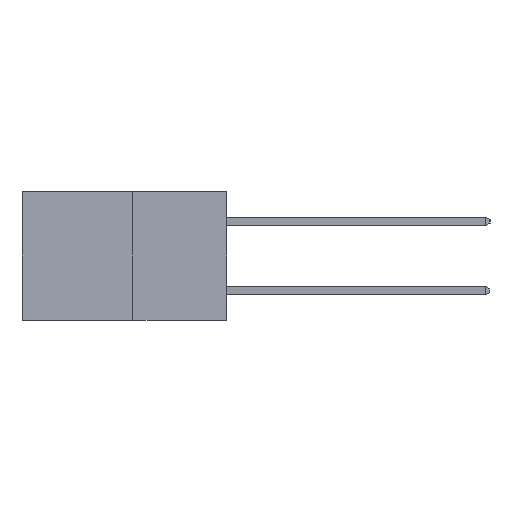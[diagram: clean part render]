
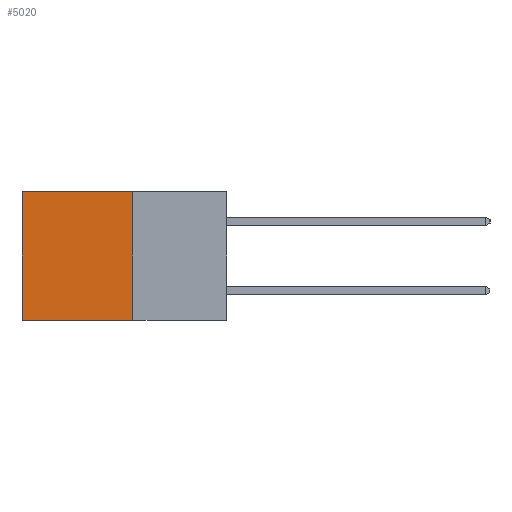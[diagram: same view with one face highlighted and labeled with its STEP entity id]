
A CAD part, left-side view. The second image highlights one B-rep face of the part: STEP entity #5020.
In plain terms, the highlighted planar face has unit normal (-1, 0, 0).
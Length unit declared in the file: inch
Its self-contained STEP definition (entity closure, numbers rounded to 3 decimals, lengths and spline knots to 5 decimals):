
#337 = FACE_OUTER_BOUND ( 'NONE', #8549, .T. ) ;
#1364 = VECTOR ( 'NONE', #9050, 39.37008 ) ;
#2038 = VECTOR ( 'NONE', #10645, 39.37008 ) ;
#2263 = VECTOR ( 'NONE', #2567, 39.37008 ) ;
#2410 = ORIENTED_EDGE ( 'NONE', *, *, #4633, .F. ) ;
#2483 = CARTESIAN_POINT ( 'NONE',  ( 0.277, 0.27, -0.37 ) ) ;
#2567 = DIRECTION ( 'NONE',  ( 0., 1., 0. ) ) ;
#3115 = VECTOR ( 'NONE', #6123, 39.37008 ) ;
#3955 = LINE ( 'NONE', #8151, #1364 ) ;
#4201 = CARTESIAN_POINT ( 'NONE',  ( 0.277, 0.27, -0.37 ) ) ;
#4343 = CARTESIAN_POINT ( 'NONE',  ( 0.277, 0.59, -0.37 ) ) ;
#4592 = LINE ( 'NONE', #9848, #2038 ) ;
#4633 = EDGE_CURVE ( 'NONE', #8775, #7240, #4816, .T. ) ;
#4816 = LINE ( 'NONE', #9108, #2263 ) ;
#5020 = ADVANCED_FACE ( 'NONE', ( #337 ), #8831, .F. ) ;
#5266 = ORIENTED_EDGE ( 'NONE', *, *, #9625, .F. ) ;
#5929 = CARTESIAN_POINT ( 'NONE',  ( 0.277, 0.59, 0. ) ) ;
#6123 = DIRECTION ( 'NONE',  ( 0., 0., -1. ) ) ;
#6163 = DIRECTION ( 'NONE',  ( 0., 0., -1. ) ) ;
#6656 = AXIS2_PLACEMENT_3D ( 'NONE', #4201, #11314, #6163 ) ;
#7047 = CARTESIAN_POINT ( 'NONE',  ( 0.277, 0.59, -0.37 ) ) ;
#7106 = EDGE_CURVE ( 'NONE', #9163, #7240, #7883, .T. ) ;
#7186 = CARTESIAN_POINT ( 'NONE',  ( 0.277, 0.27, 0. ) ) ;
#7240 = VERTEX_POINT ( 'NONE', #4343 ) ;
#7745 = ORIENTED_EDGE ( 'NONE', *, *, #10611, .T. ) ;
#7883 = LINE ( 'NONE', #7047, #3115 ) ;
#8151 = CARTESIAN_POINT ( 'NONE',  ( 0.277, 0.27, -0.37 ) ) ;
#8549 = EDGE_LOOP ( 'NONE', ( #9500, #2410, #5266, #7745 ) ) ;
#8775 = VERTEX_POINT ( 'NONE', #2483 ) ;
#8831 = PLANE ( 'NONE',  #6656 ) ;
#9050 = DIRECTION ( 'NONE',  ( 0., 0., -1. ) ) ;
#9108 = CARTESIAN_POINT ( 'NONE',  ( 0.277, 0.27, -0.37 ) ) ;
#9163 = VERTEX_POINT ( 'NONE', #5929 ) ;
#9500 = ORIENTED_EDGE ( 'NONE', *, *, #7106, .T. ) ;
#9625 = EDGE_CURVE ( 'NONE', #10606, #8775, #3955, .T. ) ;
#9848 = CARTESIAN_POINT ( 'NONE',  ( 0.277, 0.27, 0. ) ) ;
#10606 = VERTEX_POINT ( 'NONE', #7186 ) ;
#10611 = EDGE_CURVE ( 'NONE', #10606, #9163, #4592, .T. ) ;
#10645 = DIRECTION ( 'NONE',  ( 0., 1., 0. ) ) ;
#11314 = DIRECTION ( 'NONE',  ( 1., 0., 0. ) ) ;
